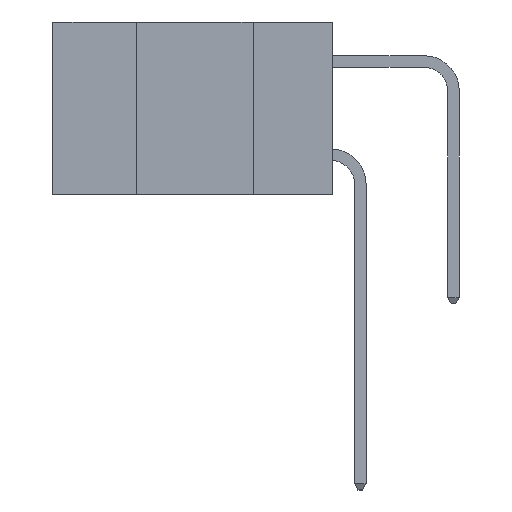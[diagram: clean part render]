
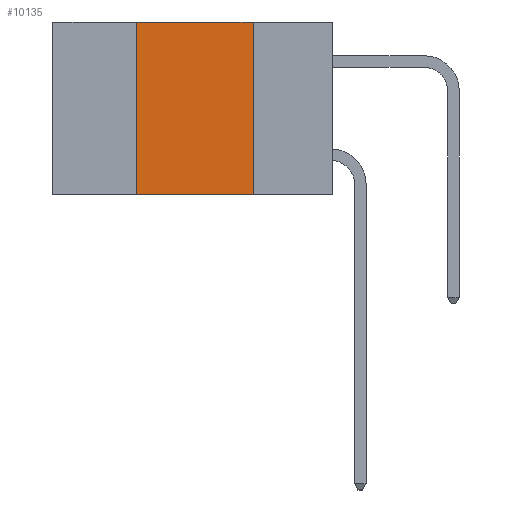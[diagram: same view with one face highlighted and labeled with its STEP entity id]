
A CAD part, left-side view. The second image highlights one B-rep face of the part: STEP entity #10135.
In plain terms, the highlighted planar face has unit normal (-1, 0, 0).
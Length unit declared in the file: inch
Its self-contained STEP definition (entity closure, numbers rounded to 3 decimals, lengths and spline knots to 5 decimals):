
#1114 = CARTESIAN_POINT ( 'NONE',  ( 0., 0.6, 0. ) ) ;
#1225 = VERTEX_POINT ( 'NONE', #4227 ) ;
#1244 = CARTESIAN_POINT ( 'NONE',  ( 0., 0.6, -0.37 ) ) ;
#1360 = DIRECTION ( 'NONE',  ( 0., 0., 1. ) ) ;
#1821 = LINE ( 'NONE', #12121, #7091 ) ;
#2203 = DIRECTION ( 'NONE',  ( 0., 0., -1. ) ) ;
#2217 = VERTEX_POINT ( 'NONE', #9137 ) ;
#2771 = VERTEX_POINT ( 'NONE', #6488 ) ;
#2975 = LINE ( 'NONE', #9535, #10290 ) ;
#3113 = VECTOR ( 'NONE', #3462, 39.37008 ) ;
#3462 = DIRECTION ( 'NONE',  ( 0., -1., 0. ) ) ;
#3610 = FACE_OUTER_BOUND ( 'NONE', #5724, .T. ) ;
#4227 = CARTESIAN_POINT ( 'NONE',  ( 0., 0.42, 0. ) ) ;
#5724 = EDGE_LOOP ( 'NONE', ( #6887, #8075, #7282, #7305 ) ) ;
#5794 = EDGE_CURVE ( 'NONE', #7646, #2217, #1821, .T. ) ;
#6488 = CARTESIAN_POINT ( 'NONE',  ( 0., 0.42, -0.37 ) ) ;
#6795 = CARTESIAN_POINT ( 'NONE',  ( 0., 0.6, 0. ) ) ;
#6887 = ORIENTED_EDGE ( 'NONE', *, *, #5794, .F. ) ;
#7091 = VECTOR ( 'NONE', #13021, 39.37008 ) ;
#7182 = EDGE_CURVE ( 'NONE', #1225, #7646, #9875, .T. ) ;
#7282 = ORIENTED_EDGE ( 'NONE', *, *, #7830, .F. ) ;
#7305 = ORIENTED_EDGE ( 'NONE', *, *, #8483, .T. ) ;
#7646 = VERTEX_POINT ( 'NONE', #11208 ) ;
#7830 = EDGE_CURVE ( 'NONE', #2771, #1225, #2975, .T. ) ;
#8075 = ORIENTED_EDGE ( 'NONE', *, *, #7182, .F. ) ;
#8401 = DIRECTION ( 'NONE',  ( 1., 0., 0. ) ) ;
#8483 = EDGE_CURVE ( 'NONE', #2771, #2217, #8545, .T. ) ;
#8545 = LINE ( 'NONE', #1244, #3113 ) ;
#9137 = CARTESIAN_POINT ( 'NONE',  ( 0., 0.17, -0.37 ) ) ;
#9535 = CARTESIAN_POINT ( 'NONE',  ( 0., 0.42, -0.37 ) ) ;
#9572 = VECTOR ( 'NONE', #9674, 39.37008 ) ;
#9674 = DIRECTION ( 'NONE',  ( 0., -1., 0. ) ) ;
#9875 = LINE ( 'NONE', #6795, #9572 ) ;
#10135 = ADVANCED_FACE ( 'NONE', ( #3610 ), #12107, .F. ) ;
#10196 = AXIS2_PLACEMENT_3D ( 'NONE', #1114, #8401, #2203 ) ;
#10290 = VECTOR ( 'NONE', #1360, 39.37008 ) ;
#11208 = CARTESIAN_POINT ( 'NONE',  ( 0., 0.17, 0. ) ) ;
#12107 = PLANE ( 'NONE',  #10196 ) ;
#12121 = CARTESIAN_POINT ( 'NONE',  ( 0., 0.17, -0.37 ) ) ;
#13021 = DIRECTION ( 'NONE',  ( 0., 0., -1. ) ) ;
